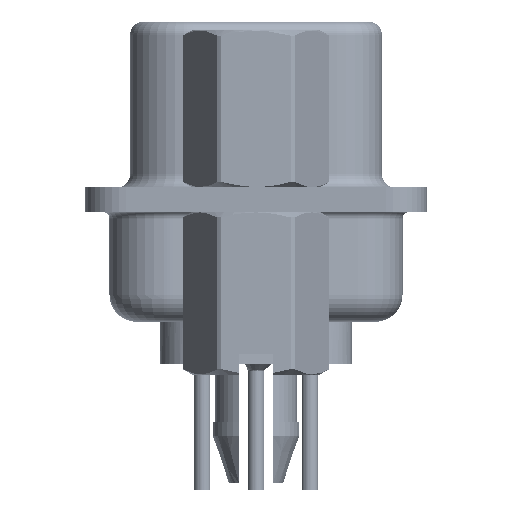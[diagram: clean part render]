
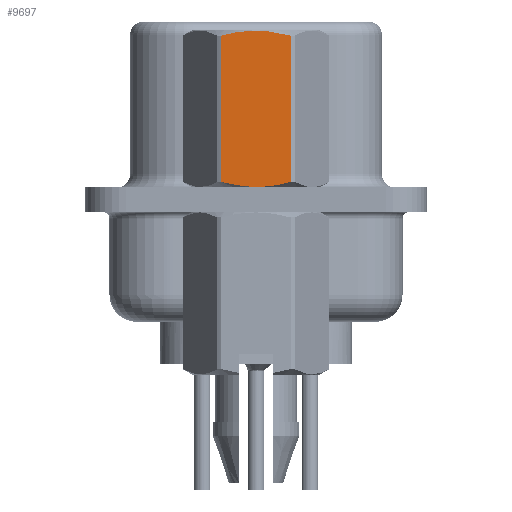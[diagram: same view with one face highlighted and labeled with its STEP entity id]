
A CAD part, left-side view. The second image highlights one B-rep face of the part: STEP entity #9697.
In plain terms, the highlighted planar face has unit normal (-1, 0, 0).
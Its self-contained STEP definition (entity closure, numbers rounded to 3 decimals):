
#245 = CARTESIAN_POINT ( 'NONE',  ( -2.381, 0.428, 0.485 ) ) ;
#412 = CARTESIAN_POINT ( 'NONE',  ( -2.381, 1.065, 0.596 ) ) ;
#897 = CARTESIAN_POINT ( 'NONE',  ( -2.381, 1.273, 3.792 ) ) ;
#1582 = CARTESIAN_POINT ( 'NONE',  ( -2.381, -1.273, 6.048 ) ) ;
#2363 = ORIENTED_EDGE ( 'NONE', *, *, #27594, .T. ) ;
#2429 = VERTEX_POINT ( 'NONE', #5290 ) ;
#3220 = EDGE_LOOP ( 'NONE', ( #4077, #24061, #2363, #31383 ) ) ;
#3409 = DIRECTION ( 'NONE',  ( 0., -1., 0. ) ) ;
#4070 = CARTESIAN_POINT ( 'NONE',  ( -2.381, 1.273, 6.048 ) ) ;
#4077 = ORIENTED_EDGE ( 'NONE', *, *, #18887, .T. ) ;
#4802 = CARTESIAN_POINT ( 'NONE',  ( -2.381, -1.273, 0.652 ) ) ;
#5290 = CARTESIAN_POINT ( 'NONE',  ( -2.381, 1.273, 0.652 ) ) ;
#5486 = CARTESIAN_POINT ( 'NONE',  ( -2.381, -0.432, 0.485 ) ) ;
#5760 = VECTOR ( 'NONE', #16417, 1000. ) ;
#7008 = CARTESIAN_POINT ( 'NONE',  ( -2.381, -0.432, 6.215 ) ) ;
#8182 = CARTESIAN_POINT ( 'NONE',  ( -2.381, -0.215, 0.468 ) ) ;
#8491 = CARTESIAN_POINT ( 'NONE',  ( -2.381, 1.375, -3.75 ) ) ;
#9697 = ADVANCED_FACE ( 'NONE', ( #23840 ), #31651, .T. ) ;
#11556 = CARTESIAN_POINT ( 'NONE',  ( -2.381, -1.066, 6.104 ) ) ;
#11728 = CARTESIAN_POINT ( 'NONE',  ( -2.381, 1.065, 6.104 ) ) ;
#12483 = B_SPLINE_CURVE_WITH_KNOTS ( 'NONE', 3,
 ( #18135, #412, #31335, #245, #28474, #8182, #5486, #15608, #13241, #18300 ),
 .UNSPECIFIED., .F., .F.,
 ( 4, 2, 2, 2, 4 ),
 ( 0.003, 0.003, 0.004, 0.004, 0.005 ),
 .UNSPECIFIED. ) ;
#13241 = CARTESIAN_POINT ( 'NONE',  ( -2.381, -1.066, 0.596 ) ) ;
#14747 = CARTESIAN_POINT ( 'NONE',  ( -2.381, 0.215, 6.232 ) ) ;
#15516 = B_SPLINE_CURVE_WITH_KNOTS ( 'NONE', 3,
 ( #30162, #11556, #22012, #7008, #19490, #14747, #25070, #16960, #11728, #32353 ),
 .UNSPECIFIED., .F., .F.,
 ( 4, 2, 2, 2, 4 ),
 ( 0.001, 0.002, 0.002, 0.003, 0.004 ),
 .UNSPECIFIED. ) ;
#15608 = CARTESIAN_POINT ( 'NONE',  ( -2.381, -0.858, 0.55 ) ) ;
#16417 = DIRECTION ( 'NONE',  ( 0., 0., -1. ) ) ;
#16960 = CARTESIAN_POINT ( 'NONE',  ( -2.381, 0.853, 6.151 ) ) ;
#18135 = CARTESIAN_POINT ( 'NONE',  ( -2.381, 1.273, 0.652 ) ) ;
#18300 = CARTESIAN_POINT ( 'NONE',  ( -2.381, -1.273, 0.652 ) ) ;
#18887 = EDGE_CURVE ( 'NONE', #2429, #23989, #12483, .T. ) ;
#19490 = CARTESIAN_POINT ( 'NONE',  ( -2.381, -0.215, 6.232 ) ) ;
#20390 = CARTESIAN_POINT ( 'NONE',  ( -2.381, -1.273, 3.792 ) ) ;
#21486 = LINE ( 'NONE', #897, #5760 ) ;
#22012 = CARTESIAN_POINT ( 'NONE',  ( -2.381, -0.858, 6.15 ) ) ;
#23840 = FACE_OUTER_BOUND ( 'NONE', #3220, .T. ) ;
#23989 = VERTEX_POINT ( 'NONE', #4802 ) ;
#24061 = ORIENTED_EDGE ( 'NONE', *, *, #25603, .T. ) ;
#25070 = CARTESIAN_POINT ( 'NONE',  ( -2.381, 0.428, 6.215 ) ) ;
#25603 = EDGE_CURVE ( 'NONE', #23989, #31251, #25628, .T. ) ;
#25628 = LINE ( 'NONE', #20390, #26700 ) ;
#26116 = DIRECTION ( 'NONE',  ( 0., 0., 1. ) ) ;
#26544 = DIRECTION ( 'NONE',  ( -1., 0., 0. ) ) ;
#26700 = VECTOR ( 'NONE', #26116, 1000. ) ;
#27594 = EDGE_CURVE ( 'NONE', #31251, #31577, #15516, .T. ) ;
#27830 = EDGE_CURVE ( 'NONE', #31577, #2429, #21486, .T. ) ;
#28474 = CARTESIAN_POINT ( 'NONE',  ( -2.381, 0.215, 0.468 ) ) ;
#28555 = AXIS2_PLACEMENT_3D ( 'NONE', #8491, #26544, #3409 ) ;
#30162 = CARTESIAN_POINT ( 'NONE',  ( -2.381, -1.273, 6.048 ) ) ;
#31251 = VERTEX_POINT ( 'NONE', #1582 ) ;
#31335 = CARTESIAN_POINT ( 'NONE',  ( -2.381, 0.853, 0.549 ) ) ;
#31383 = ORIENTED_EDGE ( 'NONE', *, *, #27830, .T. ) ;
#31577 = VERTEX_POINT ( 'NONE', #4070 ) ;
#31651 = PLANE ( 'NONE',  #28555 ) ;
#32353 = CARTESIAN_POINT ( 'NONE',  ( -2.381, 1.273, 6.048 ) ) ;
